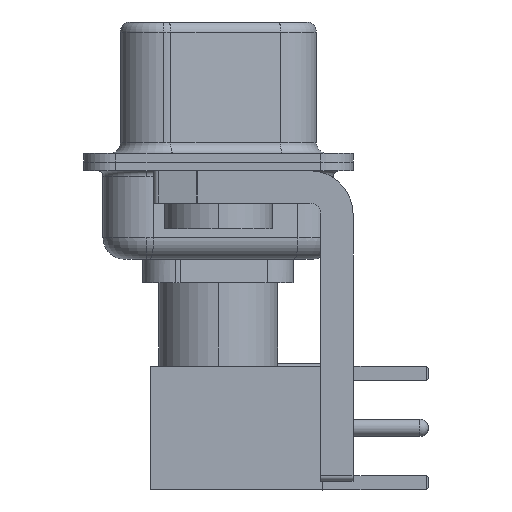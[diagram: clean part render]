
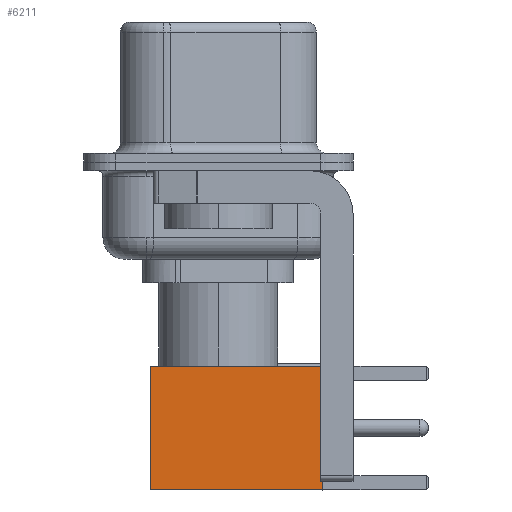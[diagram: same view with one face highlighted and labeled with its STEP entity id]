
A CAD part, left-side view. The second image highlights one B-rep face of the part: STEP entity #6211.
In plain terms, the highlighted face is planar.
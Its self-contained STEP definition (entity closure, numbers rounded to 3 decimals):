
#1749 = ORIENTED_EDGE ( 'NONE', *, *, #9889, .T. ) ;
#3289 = EDGE_CURVE ( 'NONE', #18479, #26087, #26227, .T. ) ;
#6211 = ADVANCED_FACE ( 'NONE', ( #25999 ), #30818, .T. ) ;
#6246 = CARTESIAN_POINT ( 'NONE',  ( 2.875, 2.875, 0. ) ) ;
#6579 = ORIENTED_EDGE ( 'NONE', *, *, #29712, .T. ) ;
#6722 = DIRECTION ( 'NONE',  ( 0., 0., -1. ) ) ;
#6825 = ORIENTED_EDGE ( 'NONE', *, *, #3289, .F. ) ;
#9119 = LINE ( 'NONE', #6246, #26936 ) ;
#9885 = EDGE_LOOP ( 'NONE', ( #1749, #6579, #6825, #11833 ) ) ;
#9889 = EDGE_CURVE ( 'NONE', #27987, #25433, #9119, .T. ) ;
#9942 = DIRECTION ( 'NONE',  ( -1., 0., 0. ) ) ;
#10254 = CARTESIAN_POINT ( 'NONE',  ( 0., 2.875, 0. ) ) ;
#10413 = LINE ( 'NONE', #10254, #29498 ) ;
#11569 = CARTESIAN_POINT ( 'NONE',  ( -2.875, 2.875, 8. ) ) ;
#11595 = CARTESIAN_POINT ( 'NONE',  ( -2.875, 2.875, 0. ) ) ;
#11833 = ORIENTED_EDGE ( 'NONE', *, *, #22638, .F. ) ;
#16797 = DIRECTION ( 'NONE',  ( 0., 1., 0. ) ) ;
#17882 = CARTESIAN_POINT ( 'NONE',  ( 0., 2.875, 8. ) ) ;
#18479 = VERTEX_POINT ( 'NONE', #11569 ) ;
#18571 = CARTESIAN_POINT ( 'NONE',  ( 2.875, 2.875, 0. ) ) ;
#21045 = VECTOR ( 'NONE', #27721, 1000. ) ;
#21482 = DIRECTION ( 'NONE',  ( 0., 0., 1. ) ) ;
#22638 = EDGE_CURVE ( 'NONE', #27987, #18479, #25461, .T. ) ;
#25433 = VERTEX_POINT ( 'NONE', #29947 ) ;
#25461 = LINE ( 'NONE', #17882, #21045 ) ;
#25999 = FACE_OUTER_BOUND ( 'NONE', #9885, .T. ) ;
#26087 = VERTEX_POINT ( 'NONE', #11595 ) ;
#26227 = LINE ( 'NONE', #29114, #29530 ) ;
#26386 = DIRECTION ( 'NONE',  ( 0., 0., -1. ) ) ;
#26936 = VECTOR ( 'NONE', #6722, 1000. ) ;
#27721 = DIRECTION ( 'NONE',  ( -1., 0., 0. ) ) ;
#27987 = VERTEX_POINT ( 'NONE', #30417 ) ;
#28922 = AXIS2_PLACEMENT_3D ( 'NONE', #18571, #16797, #21482 ) ;
#29114 = CARTESIAN_POINT ( 'NONE',  ( -2.875, 2.875, 0. ) ) ;
#29498 = VECTOR ( 'NONE', #9942, 1000. ) ;
#29530 = VECTOR ( 'NONE', #26386, 1000. ) ;
#29712 = EDGE_CURVE ( 'NONE', #25433, #26087, #10413, .T. ) ;
#29947 = CARTESIAN_POINT ( 'NONE',  ( 2.875, 2.875, 0. ) ) ;
#30417 = CARTESIAN_POINT ( 'NONE',  ( 2.875, 2.875, 8. ) ) ;
#30818 = PLANE ( 'NONE',  #28922 ) ;
